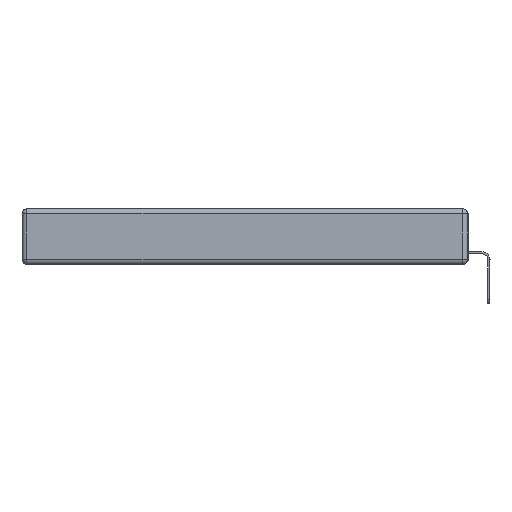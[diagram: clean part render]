
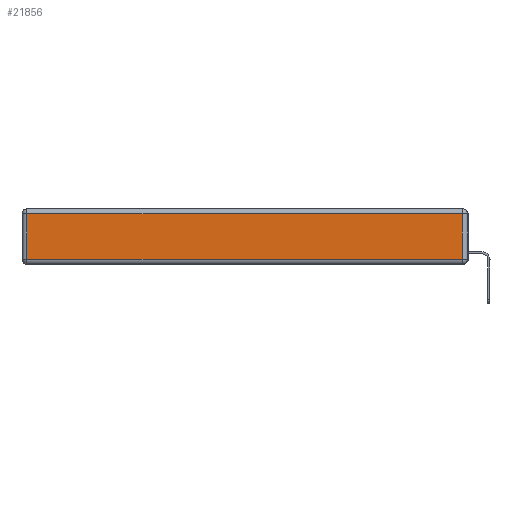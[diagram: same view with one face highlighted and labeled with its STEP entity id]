
A CAD part, left-side view. The second image highlights one B-rep face of the part: STEP entity #21856.
In plain terms, the highlighted planar face has unit normal (-1, 0, 0).
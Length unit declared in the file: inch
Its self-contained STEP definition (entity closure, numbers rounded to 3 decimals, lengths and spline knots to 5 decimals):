
#184 = VECTOR ( 'NONE', #13935, 39.37008 ) ;
#453 = DIRECTION ( 'NONE',  ( -1., 0., 0. ) ) ;
#717 = LINE ( 'NONE', #2029, #184 ) ;
#1009 = CARTESIAN_POINT ( 'NONE',  ( 0., 2.72, -0.313 ) ) ;
#1557 = EDGE_CURVE ( 'NONE', #9118, #19344, #10923, .T. ) ;
#1994 = CARTESIAN_POINT ( 'NONE',  ( 0., 0.03, -0.343 ) ) ;
#2029 = CARTESIAN_POINT ( 'NONE',  ( 0., 2.72, -0.343 ) ) ;
#2399 = CARTESIAN_POINT ( 'NONE',  ( 0., 0., -0.313 ) ) ;
#3141 = VECTOR ( 'NONE', #15824, 39.37008 ) ;
#3368 = AXIS2_PLACEMENT_3D ( 'NONE', #9000, #453, #10646 ) ;
#5460 = ORIENTED_EDGE ( 'NONE', *, *, #13691, .T. ) ;
#7065 = CARTESIAN_POINT ( 'NONE',  ( 0., 0.03, -0.03 ) ) ;
#7138 = CARTESIAN_POINT ( 'NONE',  ( 0., 2.72, -0.03 ) ) ;
#7209 = VECTOR ( 'NONE', #20683, 39.37008 ) ;
#8526 = EDGE_CURVE ( 'NONE', #21562, #9118, #19831, .T. ) ;
#8718 = ORIENTED_EDGE ( 'NONE', *, *, #19512, .T. ) ;
#8914 = CARTESIAN_POINT ( 'NONE',  ( 0., 2.75, -0.03 ) ) ;
#8989 = CARTESIAN_POINT ( 'NONE',  ( 0., 0.03, -0.313 ) ) ;
#9000 = CARTESIAN_POINT ( 'NONE',  ( 0., 0., -0.343 ) ) ;
#9118 = VERTEX_POINT ( 'NONE', #8989 ) ;
#9161 = DIRECTION ( 'NONE',  ( 0., -1., 0. ) ) ;
#10646 = DIRECTION ( 'NONE',  ( 0., 0., 1. ) ) ;
#10923 = LINE ( 'NONE', #1994, #7209 ) ;
#11954 = ORIENTED_EDGE ( 'NONE', *, *, #8526, .T. ) ;
#13691 = EDGE_CURVE ( 'NONE', #18847, #21562, #717, .T. ) ;
#13935 = DIRECTION ( 'NONE',  ( 0., 0., -1. ) ) ;
#15633 = FACE_OUTER_BOUND ( 'NONE', #16009, .T. ) ;
#15770 = PLANE ( 'NONE',  #3368 ) ;
#15824 = DIRECTION ( 'NONE',  ( 0., 1., 0. ) ) ;
#16009 = EDGE_LOOP ( 'NONE', ( #11954, #17260, #8718, #5460 ) ) ;
#17260 = ORIENTED_EDGE ( 'NONE', *, *, #1557, .T. ) ;
#18847 = VERTEX_POINT ( 'NONE', #7138 ) ;
#19344 = VERTEX_POINT ( 'NONE', #7065 ) ;
#19512 = EDGE_CURVE ( 'NONE', #19344, #18847, #19845, .T. ) ;
#19831 = LINE ( 'NONE', #2399, #21958 ) ;
#19845 = LINE ( 'NONE', #8914, #3141 ) ;
#20683 = DIRECTION ( 'NONE',  ( 0., 0., 1. ) ) ;
#21562 = VERTEX_POINT ( 'NONE', #1009 ) ;
#21856 = ADVANCED_FACE ( 'NONE', ( #15633 ), #15770, .T. ) ;
#21958 = VECTOR ( 'NONE', #9161, 39.37008 ) ;
